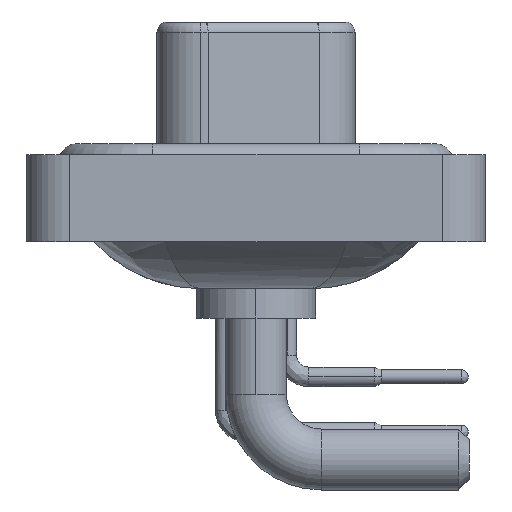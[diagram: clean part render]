
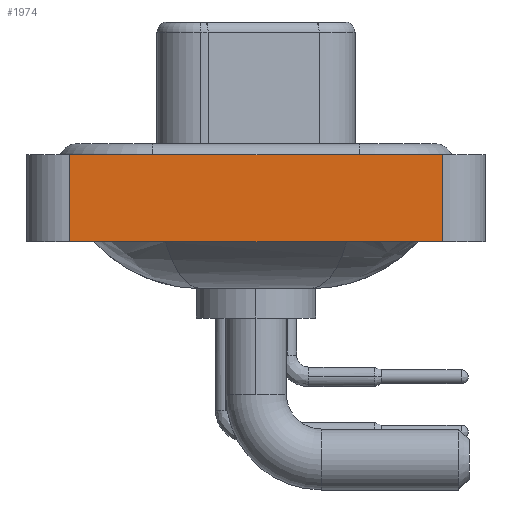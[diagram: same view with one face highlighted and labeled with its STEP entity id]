
A CAD part, left-side view. The second image highlights one B-rep face of the part: STEP entity #1974.
In plain terms, the highlighted planar face has unit normal (-1, 0, 0).
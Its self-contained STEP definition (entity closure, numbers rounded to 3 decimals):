
#614 = EDGE_CURVE ( 'NONE', #12909, #10181, #26043, .T. ) ;
#1348 = DIRECTION ( 'NONE',  ( -1., 0., 0. ) ) ;
#1958 = DIRECTION ( 'NONE',  ( 0., 0., 1. ) ) ;
#1974 = ADVANCED_FACE ( 'NONE', ( #25158 ), #26168, .T. ) ;
#3328 = CARTESIAN_POINT ( 'NONE',  ( -7.35, -8.55, -3.6 ) ) ;
#4226 = LINE ( 'NONE', #8206, #18248 ) ;
#4479 = EDGE_CURVE ( 'NONE', #10181, #15925, #4917, .T. ) ;
#4627 = VECTOR ( 'NONE', #21038, 1000. ) ;
#4917 = LINE ( 'NONE', #9399, #4627 ) ;
#6205 = VERTEX_POINT ( 'NONE', #15327 ) ;
#7140 = AXIS2_PLACEMENT_3D ( 'NONE', #3328, #1348, #7320 ) ;
#7320 = DIRECTION ( 'NONE',  ( 0., 0., 1. ) ) ;
#8206 = CARTESIAN_POINT ( 'NONE',  ( -7.35, -8.55, -3.6 ) ) ;
#8765 = ORIENTED_EDGE ( 'NONE', *, *, #19747, .T. ) ;
#9022 = ORIENTED_EDGE ( 'NONE', *, *, #23383, .T. ) ;
#9399 = CARTESIAN_POINT ( 'NONE',  ( -7.35, -8.55, 0.4 ) ) ;
#10181 = VERTEX_POINT ( 'NONE', #23986 ) ;
#12909 = VERTEX_POINT ( 'NONE', #15803 ) ;
#14187 = VECTOR ( 'NONE', #1958, 1000. ) ;
#14653 = DIRECTION ( 'NONE',  ( 0., -1., 0. ) ) ;
#15327 = CARTESIAN_POINT ( 'NONE',  ( -7.35, -8.55, -3.6 ) ) ;
#15372 = ORIENTED_EDGE ( 'NONE', *, *, #614, .F. ) ;
#15803 = CARTESIAN_POINT ( 'NONE',  ( -7.35, 8.55, -3.6 ) ) ;
#15925 = VERTEX_POINT ( 'NONE', #19733 ) ;
#17582 = CARTESIAN_POINT ( 'NONE',  ( -7.35, -8.55, -3.6 ) ) ;
#18237 = CARTESIAN_POINT ( 'NONE',  ( -7.35, 8.55, -3.6 ) ) ;
#18248 = VECTOR ( 'NONE', #14653, 1000. ) ;
#19733 = CARTESIAN_POINT ( 'NONE',  ( -7.35, -8.55, 0.4 ) ) ;
#19747 = EDGE_CURVE ( 'NONE', #12909, #6205, #4226, .T. ) ;
#20348 = EDGE_LOOP ( 'NONE', ( #9022, #23058, #15372, #8765 ) ) ;
#21038 = DIRECTION ( 'NONE',  ( 0., -1., 0. ) ) ;
#22093 = LINE ( 'NONE', #17582, #25351 ) ;
#23058 = ORIENTED_EDGE ( 'NONE', *, *, #4479, .F. ) ;
#23383 = EDGE_CURVE ( 'NONE', #6205, #15925, #22093, .T. ) ;
#23705 = DIRECTION ( 'NONE',  ( 0., 0., 1. ) ) ;
#23986 = CARTESIAN_POINT ( 'NONE',  ( -7.35, 8.55, 0.4 ) ) ;
#25158 = FACE_OUTER_BOUND ( 'NONE', #20348, .T. ) ;
#25351 = VECTOR ( 'NONE', #23705, 1000. ) ;
#26043 = LINE ( 'NONE', #18237, #14187 ) ;
#26168 = PLANE ( 'NONE',  #7140 ) ;
